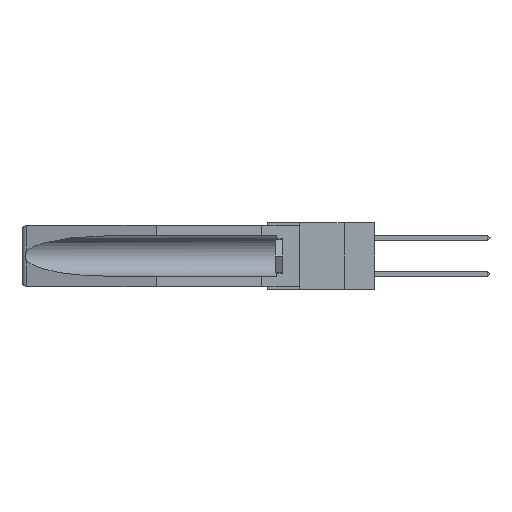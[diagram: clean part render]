
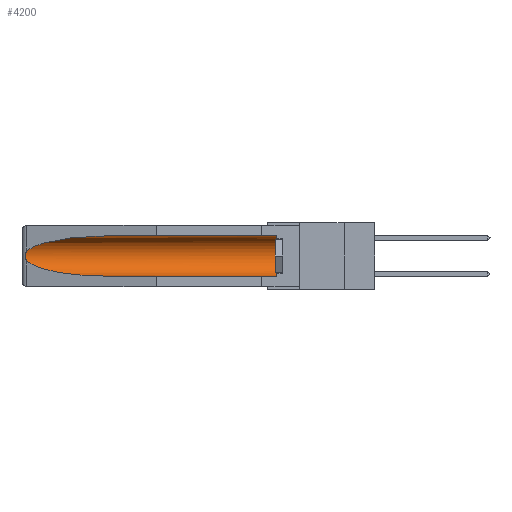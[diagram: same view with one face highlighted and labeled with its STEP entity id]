
A CAD part, left-side view. The second image highlights one B-rep face of the part: STEP entity #4200.
In plain terms, the highlighted cylindrical face has radius 2.857 mm (diameter 5.715 mm), a partial arc.
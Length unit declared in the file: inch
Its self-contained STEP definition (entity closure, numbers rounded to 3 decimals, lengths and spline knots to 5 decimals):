
#176 = CARTESIAN_POINT ( 'NONE',  ( 0.155, 1.07973, -0.284 ) ) ;
#422 = CARTESIAN_POINT ( 'NONE',  ( 0.21114, 1.30732, -0.284 ) ) ;
#829 = EDGE_CURVE ( 'NONE', #1294, #4431, #3099, .T. ) ;
#1207 = VERTEX_POINT ( 'NONE', #21655 ) ;
#1294 = VERTEX_POINT ( 'NONE', #9203 ) ;
#1367 = ORIENTED_EDGE ( 'NONE', *, *, #4996, .F. ) ;
#1991 = CARTESIAN_POINT ( 'NONE',  ( 0.26537, 1.52718, -0.19328 ) ) ;
#2486 = CARTESIAN_POINT ( 'NONE',  ( 0.26537, 1.52718, -0.14972 ) ) ;
#3099 = CIRCLE ( 'NONE', #23911, 0.1125 ) ;
#3669 = CARTESIAN_POINT ( 'NONE',  ( 0.155, -0.30754, -0.1715 ) ) ;
#3738 = VERTEX_POINT ( 'NONE', #18812 ) ;
#4009 = CARTESIAN_POINT ( 'NONE',  ( 0.2675, 1.53308, -0.16763 ) ) ;
#4200 = ADVANCED_FACE ( 'NONE', ( #5903 ), #12244, .F. ) ;
#4431 = VERTEX_POINT ( 'NONE', #10870 ) ;
#4977 = ORIENTED_EDGE ( 'NONE', *, *, #829, .T. ) ;
#4996 = EDGE_CURVE ( 'NONE', #1294, #8624, #11880, .T. ) ;
#5903 = FACE_OUTER_BOUND ( 'NONE', #23977, .T. ) ;
#6231 = CARTESIAN_POINT ( 'NONE',  ( 0.26597, 1.5296, -0.19026 ) ) ;
#7884 = EDGE_CURVE ( 'NONE', #3738, #9685, #24446, .T. ) ;
#8624 = VERTEX_POINT ( 'NONE', #176 ) ;
#9203 = CARTESIAN_POINT ( 'NONE',  ( 0.155, 0.126, -0.284 ) ) ;
#9685 = VERTEX_POINT ( 'NONE', #19457 ) ;
#9810 = ORIENTED_EDGE ( 'NONE', *, *, #26556, .T. ) ;
#10352 = CARTESIAN_POINT ( 'NONE',  ( 0.26654, 1.53092, -0.15636 ) ) ;
#10870 = CARTESIAN_POINT ( 'NONE',  ( 0.155, 0.126, -0.059 ) ) ;
#10894 = CARTESIAN_POINT ( 'NONE',  ( 0.155, 1.07973, -0.284 ) ) ;
#10940 = ORIENTED_EDGE ( 'NONE', *, *, #18400, .T. ) ;
#11036 = CARTESIAN_POINT ( 'NONE',  ( 0.21114, 1.30732, -0.059 ) ) ;
#11880 = LINE ( 'NONE', #25270, #13525 ) ;
#12244 = CYLINDRICAL_SURFACE ( 'NONE', #12818, 0.1125 ) ;
#12313 = DIRECTION ( 'NONE',  ( 0., 0., 1. ) ) ;
#12409 = B_SPLINE_CURVE_WITH_KNOTS ( 'NONE', 3,
 ( #22930, #12577, #10352, #27281, #4009, #18939, #12756, #14594, #6231, #1991 ),
 .UNSPECIFIED., .F., .F.,
 ( 4, 2, 2, 2, 4 ),
 ( 0., 0.00029, 0.00058, 0.00087, 0.00117 ),
 .UNSPECIFIED. ) ;
#12577 = CARTESIAN_POINT ( 'NONE',  ( 0.26597, 1.52961, -0.15275 ) ) ;
#12756 = CARTESIAN_POINT ( 'NONE',  ( 0.2673, 1.53269, -0.17917 ) ) ;
#12818 = AXIS2_PLACEMENT_3D ( 'NONE', #3669, #24734, #12313 ) ;
#13206 = DIRECTION ( 'NONE',  ( 0., 1., 0. ) ) ;
#13525 = VECTOR ( 'NONE', #23044, 39.37008 ) ;
#13753 = ORIENTED_EDGE ( 'NONE', *, *, #7884, .T. ) ;
#14594 = CARTESIAN_POINT ( 'NONE',  ( 0.26655, 1.53094, -0.18657 ) ) ;
#15239 = CARTESIAN_POINT ( 'NONE',  ( 0.26537, 1.52718, -0.19328 ) ) ;
#15288 = CARTESIAN_POINT ( 'NONE',  ( 0.155, 1.07973, -0.059 ) ) ;
#15333 = CARTESIAN_POINT ( 'NONE',  ( 0.25451, 1.48313, -0.24835 ) ) ;
#17077 = EDGE_CURVE ( 'NONE', #9685, #1207, #12409, .T. ) ;
#18400 = EDGE_CURVE ( 'NONE', #4431, #3738, #18707, .T. ) ;
#18707 = LINE ( 'NONE', #19774, #24684 ) ;
#18812 = CARTESIAN_POINT ( 'NONE',  ( 0.155, 1.07973, -0.059 ) ) ;
#18939 = CARTESIAN_POINT ( 'NONE',  ( 0.2675, 1.53308, -0.17534 ) ) ;
#19457 = CARTESIAN_POINT ( 'NONE',  ( 0.26537, 1.52718, -0.14972 ) ) ;
#19641 = DIRECTION ( 'NONE',  ( 0., 0., 1. ) ) ;
#19774 = CARTESIAN_POINT ( 'NONE',  ( 0.155, -0.30754, -0.059 ) ) ;
#21499 = CARTESIAN_POINT ( 'NONE',  ( 0.25451, 1.48313, -0.09465 ) ) ;
#21655 = CARTESIAN_POINT ( 'NONE',  ( 0.26537, 1.52718, -0.19328 ) ) ;
#22064 = DIRECTION ( 'NONE',  ( 0., -1., 0. ) ) ;
#22930 = CARTESIAN_POINT ( 'NONE',  ( 0.26537, 1.52718, -0.14972 ) ) ;
#23044 = DIRECTION ( 'NONE',  ( 0., 1., 0. ) ) ;
#23742 = ORIENTED_EDGE ( 'NONE', *, *, #17077, .T. ) ;
#23911 = AXIS2_PLACEMENT_3D ( 'NONE', #24111, #22064, #19641 ) ;
#23977 = EDGE_LOOP ( 'NONE', ( #13753, #23742, #9810, #1367, #4977, #10940 ) ) ;
#24111 = CARTESIAN_POINT ( 'NONE',  ( 0.155, 0.126, -0.1715 ) ) ;
#24446 =( BOUNDED_CURVE ( )  B_SPLINE_CURVE ( 3, ( #15288, #11036, #21499, #2486 ),
 .UNSPECIFIED., .F., .F. ) 
 B_SPLINE_CURVE_WITH_KNOTS ( ( 4, 4 ),
 ( 4.71239, 6.08839 ),
 .UNSPECIFIED. ) 
 CURVE ( )  GEOMETRIC_REPRESENTATION_ITEM ( )  RATIONAL_B_SPLINE_CURVE ( ( 1., 0.848, 0.848, 1. ) ) 
 REPRESENTATION_ITEM ( '' )  );
#24684 = VECTOR ( 'NONE', #13206, 39.37008 ) ;
#24734 = DIRECTION ( 'NONE',  ( 0., 1., 0. ) ) ;
#25131 =( BOUNDED_CURVE ( )  B_SPLINE_CURVE ( 3, ( #15239, #15333, #422, #10894 ),
 .UNSPECIFIED., .F., .F. ) 
 B_SPLINE_CURVE_WITH_KNOTS ( ( 4, 4 ),
 ( 0.1948, 1.5708 ),
 .UNSPECIFIED. ) 
 CURVE ( )  GEOMETRIC_REPRESENTATION_ITEM ( )  RATIONAL_B_SPLINE_CURVE ( ( 1., 0.848, 0.848, 1. ) ) 
 REPRESENTATION_ITEM ( '' )  );
#25270 = CARTESIAN_POINT ( 'NONE',  ( 0.155, -0.30754, -0.284 ) ) ;
#26556 = EDGE_CURVE ( 'NONE', #1207, #8624, #25131, .T. ) ;
#27281 = CARTESIAN_POINT ( 'NONE',  ( 0.2673, 1.5327, -0.16383 ) ) ;
